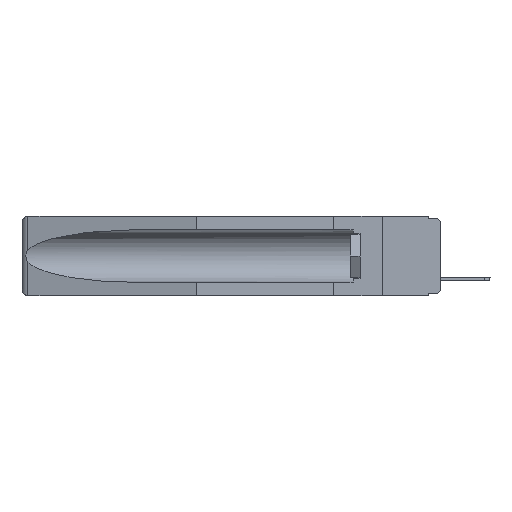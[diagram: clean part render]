
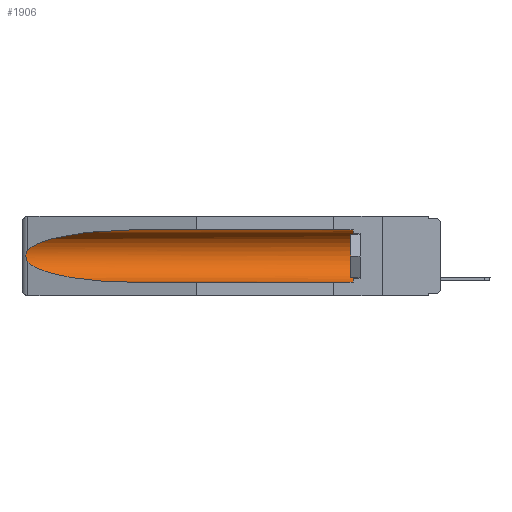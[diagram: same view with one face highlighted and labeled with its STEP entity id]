
A CAD part, left-side view. The second image highlights one B-rep face of the part: STEP entity #1906.
In plain terms, the highlighted cylindrical face has radius 2.857 mm (diameter 5.715 mm), a partial arc.
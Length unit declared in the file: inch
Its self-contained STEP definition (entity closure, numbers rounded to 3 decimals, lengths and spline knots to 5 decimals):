
#138 = CARTESIAN_POINT ( 'NONE',  ( 0.26537, 1.52718, -0.14972 ) ) ;
#347 = CARTESIAN_POINT ( 'NONE',  ( 0.155, 0.126, -0.284 ) ) ;
#1132 = ORIENTED_EDGE ( 'NONE', *, *, #10885, .T. ) ;
#1750 = CARTESIAN_POINT ( 'NONE',  ( 0.2675, 1.53308, -0.17534 ) ) ;
#1761 = VECTOR ( 'NONE', #21586, 39.37008 ) ;
#1801 = EDGE_CURVE ( 'NONE', #23540, #24764, #13565, .T. ) ;
#1900 = CYLINDRICAL_SURFACE ( 'NONE', #20973, 0.1125 ) ;
#1906 = ADVANCED_FACE ( 'NONE', ( #11574 ), #1900, .F. ) ;
#2068 = ORIENTED_EDGE ( 'NONE', *, *, #18966, .T. ) ;
#2212 = CARTESIAN_POINT ( 'NONE',  ( 0.2675, 1.53308, -0.16763 ) ) ;
#2457 = CARTESIAN_POINT ( 'NONE',  ( 0.155, -0.30754, -0.059 ) ) ;
#2717 = CARTESIAN_POINT ( 'NONE',  ( 0.155, 0.126, -0.1715 ) ) ;
#3302 =( BOUNDED_CURVE ( )  B_SPLINE_CURVE ( 3, ( #7161, #22743, #5256, #138 ),
 .UNSPECIFIED., .F., .T. ) 
 B_SPLINE_CURVE_WITH_KNOTS ( ( 4, 4 ),
 ( 4.71239, 6.08839 ),
 .UNSPECIFIED. ) 
 CURVE ( )  GEOMETRIC_REPRESENTATION_ITEM ( )  RATIONAL_B_SPLINE_CURVE ( ( 1., 0.848, 0.848, 1. ) ) 
 REPRESENTATION_ITEM ( '' )  );
#4248 = CARTESIAN_POINT ( 'NONE',  ( 0.26537, 1.52718, -0.19328 ) ) ;
#4559 = DIRECTION ( 'NONE',  ( 0., 0., 1. ) ) ;
#4624 = DIRECTION ( 'NONE',  ( 0., -1., 0. ) ) ;
#5256 = CARTESIAN_POINT ( 'NONE',  ( 0.25451, 1.48313, -0.09465 ) ) ;
#5641 = DIRECTION ( 'NONE',  ( 0., 1., 0. ) ) ;
#5959 = CARTESIAN_POINT ( 'NONE',  ( 0.26537, 1.52718, -0.19328 ) ) ;
#7061 = ORIENTED_EDGE ( 'NONE', *, *, #20890, .F. ) ;
#7161 = CARTESIAN_POINT ( 'NONE',  ( 0.155, 1.07973, -0.059 ) ) ;
#7345 = CARTESIAN_POINT ( 'NONE',  ( 0.2673, 1.5327, -0.16383 ) ) ;
#7746 = CARTESIAN_POINT ( 'NONE',  ( 0.155, 1.07973, -0.284 ) ) ;
#8535 = ORIENTED_EDGE ( 'NONE', *, *, #19155, .T. ) ;
#9214 = LINE ( 'NONE', #25045, #17669 ) ;
#9928 = CARTESIAN_POINT ( 'NONE',  ( 0.155, 0.126, -0.059 ) ) ;
#9969 = EDGE_CURVE ( 'NONE', #18603, #15367, #3302, .T. ) ;
#9973 = CARTESIAN_POINT ( 'NONE',  ( 0.2673, 1.53269, -0.17917 ) ) ;
#10014 = ORIENTED_EDGE ( 'NONE', *, *, #9969, .T. ) ;
#10885 = EDGE_CURVE ( 'NONE', #15367, #23540, #16245, .T. ) ;
#11420 = CARTESIAN_POINT ( 'NONE',  ( 0.26597, 1.5296, -0.19026 ) ) ;
#11574 = FACE_OUTER_BOUND ( 'NONE', #17420, .T. ) ;
#12395 = DIRECTION ( 'NONE',  ( 0., 0., 1. ) ) ;
#13214 = CARTESIAN_POINT ( 'NONE',  ( 0.26597, 1.52961, -0.15275 ) ) ;
#13565 =( BOUNDED_CURVE ( )  B_SPLINE_CURVE ( 3, ( #5959, #25119, #15286, #7746 ),
 .UNSPECIFIED., .F., .T. ) 
 B_SPLINE_CURVE_WITH_KNOTS ( ( 4, 4 ),
 ( 0.1948, 1.5708 ),
 .UNSPECIFIED. ) 
 CURVE ( )  GEOMETRIC_REPRESENTATION_ITEM ( )  RATIONAL_B_SPLINE_CURVE ( ( 1., 0.848, 0.848, 1. ) ) 
 REPRESENTATION_ITEM ( '' )  );
#14710 = VERTEX_POINT ( 'NONE', #9928 ) ;
#15286 = CARTESIAN_POINT ( 'NONE',  ( 0.21114, 1.30732, -0.284 ) ) ;
#15367 = VERTEX_POINT ( 'NONE', #21119 ) ;
#15607 = AXIS2_PLACEMENT_3D ( 'NONE', #2717, #4624, #12395 ) ;
#16245 = B_SPLINE_CURVE_WITH_KNOTS ( 'NONE', 3,
 ( #18979, #13214, #17183, #7345, #2212, #1750, #9973, #17306, #11420, #4248 ),
 .UNSPECIFIED., .F., .F.,
 ( 4, 2, 2, 2, 4 ),
 ( 0., 0.00029, 0.00058, 0.00087, 0.00117 ),
 .UNSPECIFIED. ) ;
#17139 = CARTESIAN_POINT ( 'NONE',  ( 0.155, 1.07973, -0.284 ) ) ;
#17183 = CARTESIAN_POINT ( 'NONE',  ( 0.26654, 1.53092, -0.15636 ) ) ;
#17306 = CARTESIAN_POINT ( 'NONE',  ( 0.26655, 1.53094, -0.18657 ) ) ;
#17324 = CARTESIAN_POINT ( 'NONE',  ( 0.155, 1.07973, -0.059 ) ) ;
#17420 = EDGE_LOOP ( 'NONE', ( #10014, #1132, #18515, #7061, #8535, #2068 ) ) ;
#17669 = VECTOR ( 'NONE', #5641, 39.37008 ) ;
#18188 = CARTESIAN_POINT ( 'NONE',  ( 0.26537, 1.52718, -0.19328 ) ) ;
#18515 = ORIENTED_EDGE ( 'NONE', *, *, #1801, .T. ) ;
#18603 = VERTEX_POINT ( 'NONE', #17324 ) ;
#18966 = EDGE_CURVE ( 'NONE', #14710, #18603, #20070, .T. ) ;
#18979 = CARTESIAN_POINT ( 'NONE',  ( 0.26537, 1.52718, -0.14972 ) ) ;
#19155 = EDGE_CURVE ( 'NONE', #22998, #14710, #19279, .T. ) ;
#19279 = CIRCLE ( 'NONE', #15607, 0.1125 ) ;
#20070 = LINE ( 'NONE', #2457, #1761 ) ;
#20890 = EDGE_CURVE ( 'NONE', #22998, #24764, #9214, .T. ) ;
#20973 = AXIS2_PLACEMENT_3D ( 'NONE', #21914, #22040, #4559 ) ;
#21119 = CARTESIAN_POINT ( 'NONE',  ( 0.26537, 1.52718, -0.14972 ) ) ;
#21586 = DIRECTION ( 'NONE',  ( 0., 1., 0. ) ) ;
#21914 = CARTESIAN_POINT ( 'NONE',  ( 0.155, -0.30754, -0.1715 ) ) ;
#22040 = DIRECTION ( 'NONE',  ( 0., 1., 0. ) ) ;
#22743 = CARTESIAN_POINT ( 'NONE',  ( 0.21114, 1.30732, -0.059 ) ) ;
#22998 = VERTEX_POINT ( 'NONE', #347 ) ;
#23540 = VERTEX_POINT ( 'NONE', #18188 ) ;
#24764 = VERTEX_POINT ( 'NONE', #17139 ) ;
#25045 = CARTESIAN_POINT ( 'NONE',  ( 0.155, -0.30754, -0.284 ) ) ;
#25119 = CARTESIAN_POINT ( 'NONE',  ( 0.25451, 1.48313, -0.24835 ) ) ;
